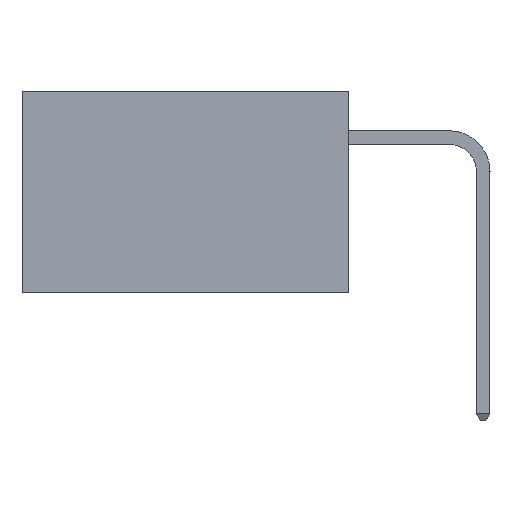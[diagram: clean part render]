
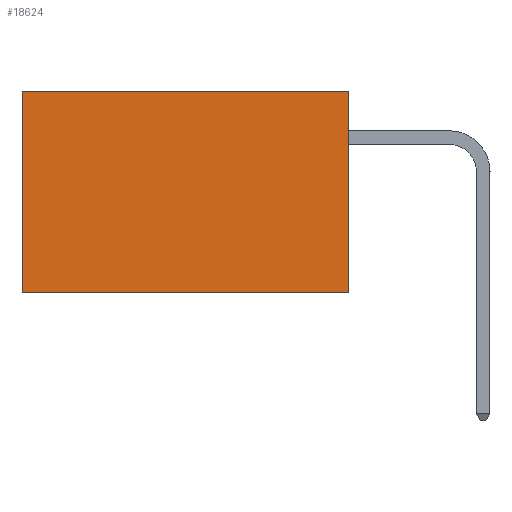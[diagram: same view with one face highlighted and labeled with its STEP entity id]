
A CAD part, left-side view. The second image highlights one B-rep face of the part: STEP entity #18624.
In plain terms, the highlighted planar face has unit normal (-1, 0, 0).
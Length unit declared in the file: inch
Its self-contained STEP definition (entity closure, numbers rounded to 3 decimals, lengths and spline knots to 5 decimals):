
#806 = LINE ( 'NONE', #14841, #7431 ) ;
#2094 = CARTESIAN_POINT ( 'NONE',  ( 0.2875, 0., 0. ) ) ;
#2333 = EDGE_CURVE ( 'NONE', #3567, #13367, #4757, .T. ) ;
#2470 = DIRECTION ( 'NONE',  ( 0., 0., -1. ) ) ;
#2501 = ORIENTED_EDGE ( 'NONE', *, *, #24495, .F. ) ;
#3558 = DIRECTION ( 'NONE',  ( 0., 1., 0. ) ) ;
#3567 = VERTEX_POINT ( 'NONE', #36560 ) ;
#4195 = CARTESIAN_POINT ( 'NONE',  ( 0.2875, 0.6, 0. ) ) ;
#4757 = LINE ( 'NONE', #2094, #26562 ) ;
#6644 = EDGE_LOOP ( 'NONE', ( #17710, #33170, #2501, #19137 ) ) ;
#7431 = VECTOR ( 'NONE', #3558, 39.37008 ) ;
#8033 = CARTESIAN_POINT ( 'NONE',  ( 0.2875, 0., 0. ) ) ;
#10216 = DIRECTION ( 'NONE',  ( 0., 0., -1. ) ) ;
#10479 = CARTESIAN_POINT ( 'NONE',  ( 0.2875, 0.6, -0.37 ) ) ;
#11248 = CARTESIAN_POINT ( 'NONE',  ( 0.2875, 0., -0.37 ) ) ;
#12785 = CARTESIAN_POINT ( 'NONE',  ( 0.2875, 0.6, 0. ) ) ;
#13058 = FACE_OUTER_BOUND ( 'NONE', #6644, .T. ) ;
#13367 = VERTEX_POINT ( 'NONE', #12785 ) ;
#13389 = VECTOR ( 'NONE', #15491, 39.37008 ) ;
#14275 = LINE ( 'NONE', #4195, #13389 ) ;
#14841 = CARTESIAN_POINT ( 'NONE',  ( 0.2875, 0., -0.37 ) ) ;
#15491 = DIRECTION ( 'NONE',  ( 0., 0., -1. ) ) ;
#17710 = ORIENTED_EDGE ( 'NONE', *, *, #21866, .T. ) ;
#18624 = ADVANCED_FACE ( 'NONE', ( #13058 ), #30894, .F. ) ;
#19137 = ORIENTED_EDGE ( 'NONE', *, *, #2333, .T. ) ;
#19488 = DIRECTION ( 'NONE',  ( 1., 0., 0. ) ) ;
#21866 = EDGE_CURVE ( 'NONE', #13367, #23918, #14275, .T. ) ;
#23452 = VERTEX_POINT ( 'NONE', #11248 ) ;
#23918 = VERTEX_POINT ( 'NONE', #10479 ) ;
#24495 = EDGE_CURVE ( 'NONE', #3567, #23452, #30629, .T. ) ;
#24748 = VECTOR ( 'NONE', #10216, 39.37008 ) ;
#26562 = VECTOR ( 'NONE', #29743, 39.37008 ) ;
#27297 = CARTESIAN_POINT ( 'NONE',  ( 0.2875, 0., 0. ) ) ;
#28239 = EDGE_CURVE ( 'NONE', #23452, #23918, #806, .T. ) ;
#29743 = DIRECTION ( 'NONE',  ( 0., 1., 0. ) ) ;
#30629 = LINE ( 'NONE', #27297, #24748 ) ;
#30894 = PLANE ( 'NONE',  #35881 ) ;
#33170 = ORIENTED_EDGE ( 'NONE', *, *, #28239, .F. ) ;
#35881 = AXIS2_PLACEMENT_3D ( 'NONE', #8033, #19488, #2470 ) ;
#36560 = CARTESIAN_POINT ( 'NONE',  ( 0.2875, 0., 0. ) ) ;
